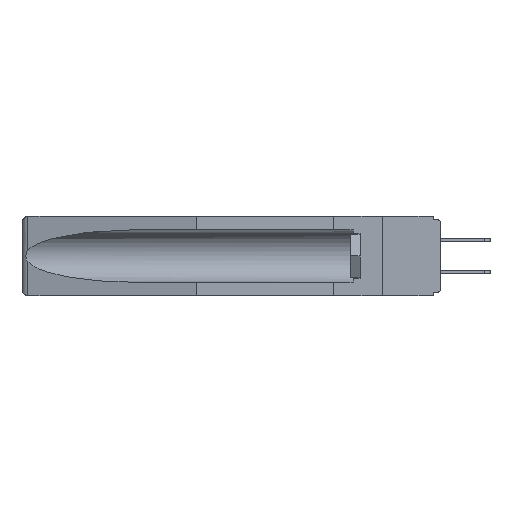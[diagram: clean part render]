
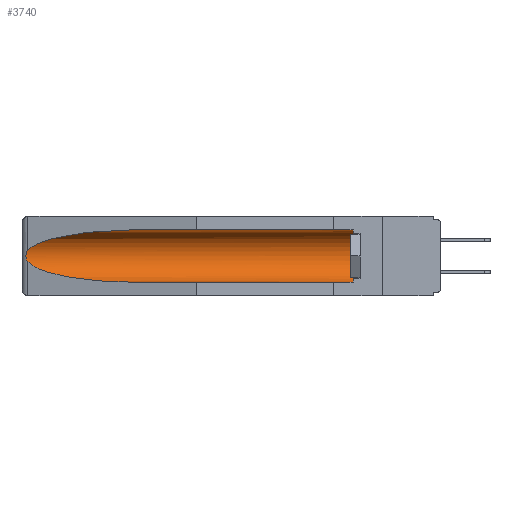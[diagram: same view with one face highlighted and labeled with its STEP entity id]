
A CAD part, left-side view. The second image highlights one B-rep face of the part: STEP entity #3740.
In plain terms, the highlighted cylindrical face has radius 2.857 mm (diameter 5.715 mm), a partial arc.
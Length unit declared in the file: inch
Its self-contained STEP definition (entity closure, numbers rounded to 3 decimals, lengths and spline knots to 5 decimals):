
#825 = DIRECTION ( 'NONE',  ( 0., 1., 0. ) ) ;
#1175 = CARTESIAN_POINT ( 'NONE',  ( 0.25451, 1.48313, -0.09465 ) ) ;
#1425 = DIRECTION ( 'NONE',  ( 0., -1., 0. ) ) ;
#2221 = EDGE_CURVE ( 'NONE', #12169, #15061, #16866, .T. ) ;
#2276 = ORIENTED_EDGE ( 'NONE', *, *, #4952, .T. ) ;
#2627 = CARTESIAN_POINT ( 'NONE',  ( 0.155, 1.07973, -0.059 ) ) ;
#3661 = CARTESIAN_POINT ( 'NONE',  ( 0.155, 0.126, -0.059 ) ) ;
#3740 = ADVANCED_FACE ( 'NONE', ( #17991 ), #16557, .F. ) ;
#4041 = CARTESIAN_POINT ( 'NONE',  ( 0.155, 1.07973, -0.059 ) ) ;
#4565 = AXIS2_PLACEMENT_3D ( 'NONE', #8946, #1425, #16895 ) ;
#4626 = CARTESIAN_POINT ( 'NONE',  ( 0.155, 1.07973, -0.284 ) ) ;
#4766 = CARTESIAN_POINT ( 'NONE',  ( 0.26597, 1.52961, -0.15275 ) ) ;
#4952 = EDGE_CURVE ( 'NONE', #6521, #5423, #10872, .T. ) ;
#5423 = VERTEX_POINT ( 'NONE', #18301 ) ;
#5604 = CARTESIAN_POINT ( 'NONE',  ( 0.21114, 1.30732, -0.059 ) ) ;
#5970 = LINE ( 'NONE', #13095, #9138 ) ;
#6048 = CARTESIAN_POINT ( 'NONE',  ( 0.155, 1.07973, -0.284 ) ) ;
#6309 = CARTESIAN_POINT ( 'NONE',  ( 0.21114, 1.30732, -0.284 ) ) ;
#6395 = CARTESIAN_POINT ( 'NONE',  ( 0.26654, 1.53092, -0.15636 ) ) ;
#6521 = VERTEX_POINT ( 'NONE', #7696 ) ;
#7086 = VECTOR ( 'NONE', #825, 39.37008 ) ;
#7105 = LINE ( 'NONE', #13226, #7086 ) ;
#7456 = CARTESIAN_POINT ( 'NONE',  ( 0.25451, 1.48313, -0.24835 ) ) ;
#7670 = CARTESIAN_POINT ( 'NONE',  ( 0.26537, 1.52718, -0.19328 ) ) ;
#7696 = CARTESIAN_POINT ( 'NONE',  ( 0.26537, 1.52718, -0.14972 ) ) ;
#7708 = CARTESIAN_POINT ( 'NONE',  ( 0.2673, 1.53269, -0.17917 ) ) ;
#7863 =( BOUNDED_CURVE ( )  B_SPLINE_CURVE ( 3, ( #7670, #7456, #6309, #6048 ),
 .UNSPECIFIED., .F., .F. ) 
 B_SPLINE_CURVE_WITH_KNOTS ( ( 4, 4 ),
 ( 0.1948, 1.5708 ),
 .UNSPECIFIED. ) 
 CURVE ( )  GEOMETRIC_REPRESENTATION_ITEM ( )  RATIONAL_B_SPLINE_CURVE ( ( 1., 0.848, 0.848, 1. ) ) 
 REPRESENTATION_ITEM ( '' )  );
#7866 = CARTESIAN_POINT ( 'NONE',  ( 0.2675, 1.53308, -0.17534 ) ) ;
#8645 = CARTESIAN_POINT ( 'NONE',  ( 0.155, -0.30754, -0.1715 ) ) ;
#8946 = CARTESIAN_POINT ( 'NONE',  ( 0.155, 0.126, -0.1715 ) ) ;
#9080 = ORIENTED_EDGE ( 'NONE', *, *, #2221, .T. ) ;
#9138 = VECTOR ( 'NONE', #13280, 39.37008 ) ;
#9155 = EDGE_CURVE ( 'NONE', #12169, #19689, #5970, .T. ) ;
#9579 = CARTESIAN_POINT ( 'NONE',  ( 0.26655, 1.53094, -0.18657 ) ) ;
#9745 = EDGE_CURVE ( 'NONE', #17647, #6521, #16571, .T. ) ;
#10872 = B_SPLINE_CURVE_WITH_KNOTS ( 'NONE', 3,
 ( #15745, #4766, #6395, #17170, #17037, #7866, #7708, #9579, #18531, #18679 ),
 .UNSPECIFIED., .F., .F.,
 ( 4, 2, 2, 2, 4 ),
 ( 0., 0.00029, 0.00058, 0.00087, 0.00117 ),
 .UNSPECIFIED. ) ;
#11129 = EDGE_LOOP ( 'NONE', ( #14521, #2276, #12394, #15252, #9080, #16226 ) ) ;
#11741 = DIRECTION ( 'NONE',  ( 0., 1., 0. ) ) ;
#12169 = VERTEX_POINT ( 'NONE', #17370 ) ;
#12201 = EDGE_CURVE ( 'NONE', #15061, #17647, #7105, .T. ) ;
#12394 = ORIENTED_EDGE ( 'NONE', *, *, #15553, .T. ) ;
#13095 = CARTESIAN_POINT ( 'NONE',  ( 0.155, -0.30754, -0.284 ) ) ;
#13226 = CARTESIAN_POINT ( 'NONE',  ( 0.155, -0.30754, -0.059 ) ) ;
#13280 = DIRECTION ( 'NONE',  ( 0., 1., 0. ) ) ;
#14521 = ORIENTED_EDGE ( 'NONE', *, *, #9745, .T. ) ;
#14845 = DIRECTION ( 'NONE',  ( 0., 0., 1. ) ) ;
#15061 = VERTEX_POINT ( 'NONE', #3661 ) ;
#15252 = ORIENTED_EDGE ( 'NONE', *, *, #9155, .F. ) ;
#15553 = EDGE_CURVE ( 'NONE', #5423, #19689, #7863, .T. ) ;
#15745 = CARTESIAN_POINT ( 'NONE',  ( 0.26537, 1.52718, -0.14972 ) ) ;
#16226 = ORIENTED_EDGE ( 'NONE', *, *, #12201, .T. ) ;
#16525 = CARTESIAN_POINT ( 'NONE',  ( 0.26537, 1.52718, -0.14972 ) ) ;
#16557 = CYLINDRICAL_SURFACE ( 'NONE', #18421, 0.1125 ) ;
#16571 =( BOUNDED_CURVE ( )  B_SPLINE_CURVE ( 3, ( #2627, #5604, #1175, #16525 ),
 .UNSPECIFIED., .F., .F. ) 
 B_SPLINE_CURVE_WITH_KNOTS ( ( 4, 4 ),
 ( 4.71239, 6.08839 ),
 .UNSPECIFIED. ) 
 CURVE ( )  GEOMETRIC_REPRESENTATION_ITEM ( )  RATIONAL_B_SPLINE_CURVE ( ( 1., 0.848, 0.848, 1. ) ) 
 REPRESENTATION_ITEM ( '' )  );
#16866 = CIRCLE ( 'NONE', #4565, 0.1125 ) ;
#16895 = DIRECTION ( 'NONE',  ( 0., 0., 1. ) ) ;
#17037 = CARTESIAN_POINT ( 'NONE',  ( 0.2675, 1.53308, -0.16763 ) ) ;
#17170 = CARTESIAN_POINT ( 'NONE',  ( 0.2673, 1.5327, -0.16383 ) ) ;
#17370 = CARTESIAN_POINT ( 'NONE',  ( 0.155, 0.126, -0.284 ) ) ;
#17647 = VERTEX_POINT ( 'NONE', #4041 ) ;
#17991 = FACE_OUTER_BOUND ( 'NONE', #11129, .T. ) ;
#18301 = CARTESIAN_POINT ( 'NONE',  ( 0.26537, 1.52718, -0.19328 ) ) ;
#18421 = AXIS2_PLACEMENT_3D ( 'NONE', #8645, #11741, #14845 ) ;
#18531 = CARTESIAN_POINT ( 'NONE',  ( 0.26597, 1.5296, -0.19026 ) ) ;
#18679 = CARTESIAN_POINT ( 'NONE',  ( 0.26537, 1.52718, -0.19328 ) ) ;
#19689 = VERTEX_POINT ( 'NONE', #4626 ) ;
